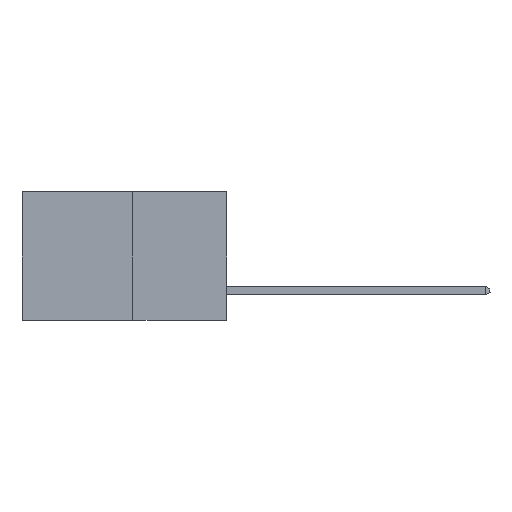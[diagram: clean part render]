
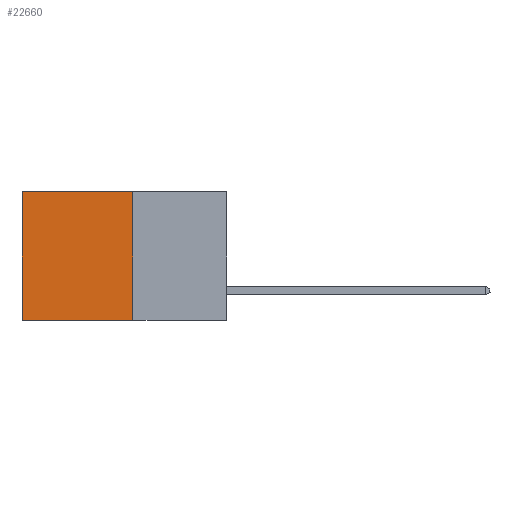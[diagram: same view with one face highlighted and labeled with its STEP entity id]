
A CAD part, left-side view. The second image highlights one B-rep face of the part: STEP entity #22660.
In plain terms, the highlighted planar face has unit normal (-1, 0, 0).
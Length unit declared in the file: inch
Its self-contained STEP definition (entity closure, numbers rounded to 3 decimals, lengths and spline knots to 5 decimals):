
#1798 = EDGE_CURVE ( 'NONE', #15486, #17054, #10638, .T. ) ;
#2260 = DIRECTION ( 'NONE',  ( 0., 0., -1. ) ) ;
#2525 = CARTESIAN_POINT ( 'NONE',  ( 0.277, 0.59, -0.37 ) ) ;
#2843 = EDGE_LOOP ( 'NONE', ( #14276, #20202, #11056, #17381 ) ) ;
#4642 = FACE_OUTER_BOUND ( 'NONE', #2843, .T. ) ;
#5508 = VECTOR ( 'NONE', #11183, 39.37008 ) ;
#6084 = CARTESIAN_POINT ( 'NONE',  ( 0.277, 0.27, -0.37 ) ) ;
#6408 = CARTESIAN_POINT ( 'NONE',  ( 0.277, 0.59, 0. ) ) ;
#7167 = VERTEX_POINT ( 'NONE', #10326 ) ;
#8415 = VECTOR ( 'NONE', #20059, 39.37008 ) ;
#10326 = CARTESIAN_POINT ( 'NONE',  ( 0.277, 0.27, 0. ) ) ;
#10555 = CARTESIAN_POINT ( 'NONE',  ( 0.277, 0.27, -0.37 ) ) ;
#10638 = LINE ( 'NONE', #2525, #5508 ) ;
#11056 = ORIENTED_EDGE ( 'NONE', *, *, #15863, .F. ) ;
#11183 = DIRECTION ( 'NONE',  ( 0., 0., -1. ) ) ;
#11890 = PLANE ( 'NONE',  #18878 ) ;
#12313 = VERTEX_POINT ( 'NONE', #13936 ) ;
#13048 = CARTESIAN_POINT ( 'NONE',  ( 0.277, 0.59, -0.37 ) ) ;
#13118 = CARTESIAN_POINT ( 'NONE',  ( 0.277, 0.27, 0. ) ) ;
#13188 = VECTOR ( 'NONE', #21232, 39.37008 ) ;
#13813 = DIRECTION ( 'NONE',  ( 1., 0., 0. ) ) ;
#13936 = CARTESIAN_POINT ( 'NONE',  ( 0.277, 0.27, -0.37 ) ) ;
#14276 = ORIENTED_EDGE ( 'NONE', *, *, #1798, .T. ) ;
#14849 = VECTOR ( 'NONE', #18868, 39.37008 ) ;
#15044 = EDGE_CURVE ( 'NONE', #12313, #17054, #17980, .T. ) ;
#15486 = VERTEX_POINT ( 'NONE', #6408 ) ;
#15863 = EDGE_CURVE ( 'NONE', #7167, #12313, #23302, .T. ) ;
#17054 = VERTEX_POINT ( 'NONE', #13048 ) ;
#17381 = ORIENTED_EDGE ( 'NONE', *, *, #23070, .T. ) ;
#17455 = CARTESIAN_POINT ( 'NONE',  ( 0.277, 0.27, -0.37 ) ) ;
#17980 = LINE ( 'NONE', #10555, #8415 ) ;
#18868 = DIRECTION ( 'NONE',  ( 0., 1., 0. ) ) ;
#18878 = AXIS2_PLACEMENT_3D ( 'NONE', #6084, #13813, #2260 ) ;
#19901 = LINE ( 'NONE', #13118, #14849 ) ;
#20059 = DIRECTION ( 'NONE',  ( 0., 1., 0. ) ) ;
#20202 = ORIENTED_EDGE ( 'NONE', *, *, #15044, .F. ) ;
#21232 = DIRECTION ( 'NONE',  ( 0., 0., -1. ) ) ;
#22660 = ADVANCED_FACE ( 'NONE', ( #4642 ), #11890, .F. ) ;
#23070 = EDGE_CURVE ( 'NONE', #7167, #15486, #19901, .T. ) ;
#23302 = LINE ( 'NONE', #17455, #13188 ) ;
